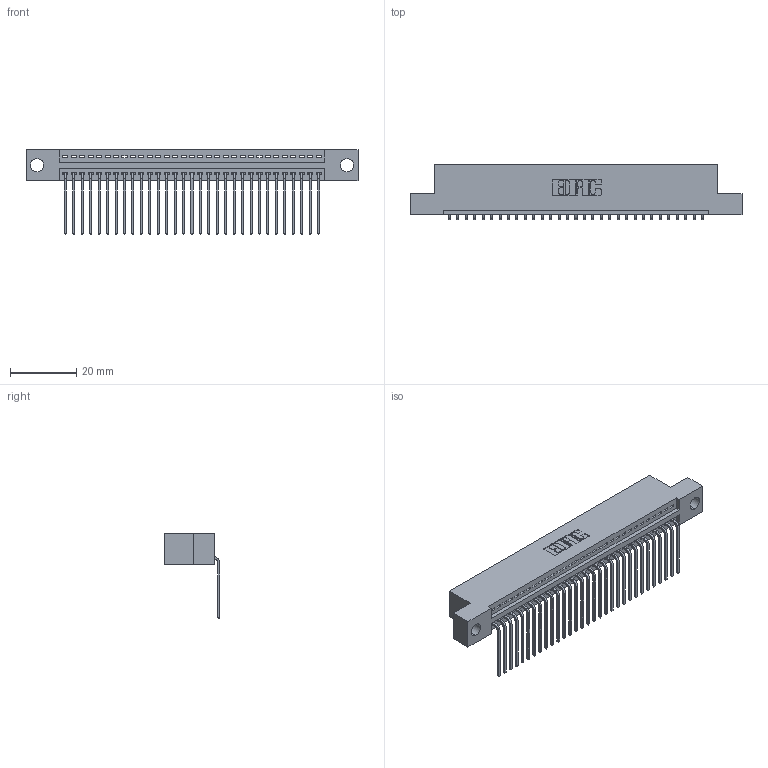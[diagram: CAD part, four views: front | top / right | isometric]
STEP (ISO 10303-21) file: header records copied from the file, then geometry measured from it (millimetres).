
FILE_DESCRIPTION (( 'STEP AP203' ), '1' );
FILE_NAME ('345-031-559-104.STEP', '2018-08-23T12:00:18', ( '' ), ( '' ), 'SwSTEP 2.0', 'SolidWorks 2016', '' );
FILE_SCHEMA (( 'CONFIG_CONTROL_DESIGN' ));
Length unit declared in the file: inch
Products named in the file (3): 345 Part_Flush Mounting Lugs - 0.156 Dia-TH; 345-292-001_558 559 Tail - 1; 345-031-559-104
Assembly tree (32 placements, depth 2):
  345-031-559-104
    345 Part_Flush Mounting Lugs - 0.156 Dia-TH
    345-292-001_558 559 Tail - 1  x31
Bounding box: 99.95 x 16.75 x 25.53 mm (x, y, z)
Volume: 9418.6 mm3; surface area: 12782.6 mm2
Topology: 32 solids, 32 shells, 1986 faces, 5983 edges, 3946 vertices
Faces by surface type: plane 1382, cylinder 604
Entity records: 24899 total; most frequent: CARTESIAN_POINT 4321, ORIENTED_EDGE 4286, DIRECTION 3789, EDGE_CURVE 2143, LINE 1887, VECTOR 1887, VERTEX_POINT 1426, AXIS2_PLACEMENT_3D 951
